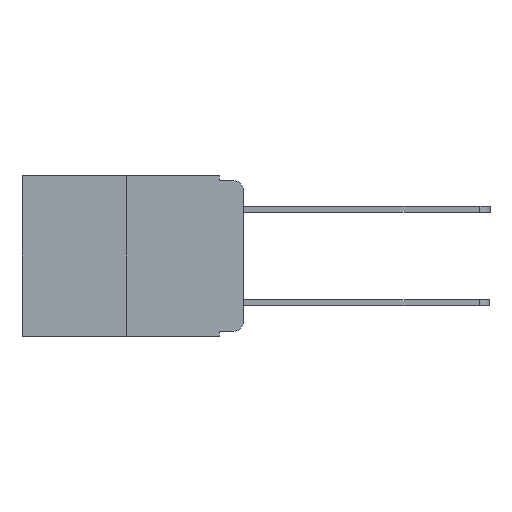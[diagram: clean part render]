
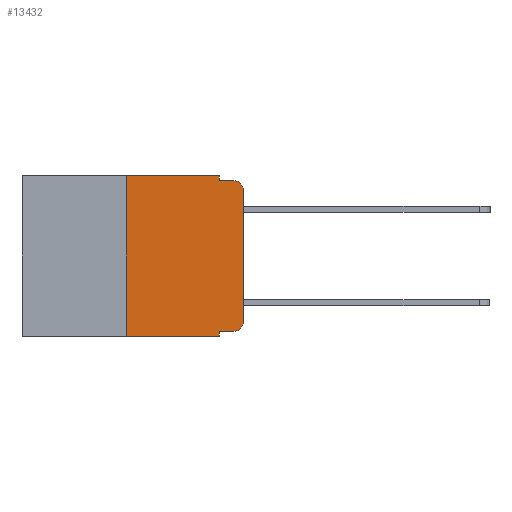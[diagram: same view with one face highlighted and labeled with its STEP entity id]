
A CAD part, left-side view. The second image highlights one B-rep face of the part: STEP entity #13432.
In plain terms, the highlighted planar face has unit normal (-1, 0, 0).
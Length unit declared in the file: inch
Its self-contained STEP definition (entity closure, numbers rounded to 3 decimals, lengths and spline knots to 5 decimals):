
#126 = CARTESIAN_POINT ( 'NONE',  ( 0., 0.051, -0.343 ) ) ;
#410 = PLANE ( 'NONE',  #3341 ) ;
#435 = EDGE_CURVE ( 'NONE', #3251, #18637, #3825, .T. ) ;
#1491 = AXIS2_PLACEMENT_3D ( 'NONE', #7417, #7707, #7675 ) ;
#1815 = EDGE_CURVE ( 'NONE', #4663, #12088, #8660, .T. ) ;
#2210 = ORIENTED_EDGE ( 'NONE', *, *, #16000, .F. ) ;
#2294 = CARTESIAN_POINT ( 'NONE',  ( 0., 0.473, 0. ) ) ;
#2514 = VECTOR ( 'NONE', #19189, 39.37008 ) ;
#3236 = LINE ( 'NONE', #6667, #21598 ) ;
#3251 = VERTEX_POINT ( 'NONE', #10124 ) ;
#3277 = DIRECTION ( 'NONE',  ( 0., 0., -1. ) ) ;
#3341 = AXIS2_PLACEMENT_3D ( 'NONE', #2294, #5998, #18486 ) ;
#3568 = FACE_OUTER_BOUND ( 'NONE', #18751, .T. ) ;
#3825 = LINE ( 'NONE', #6593, #17067 ) ;
#3938 = CARTESIAN_POINT ( 'NONE',  ( 0., 0.25, -0.343 ) ) ;
#4457 = CARTESIAN_POINT ( 'NONE',  ( 0., 0., -0.03 ) ) ;
#4663 = VERTEX_POINT ( 'NONE', #3938 ) ;
#4794 = EDGE_CURVE ( 'NONE', #7147, #11658, #18959, .T. ) ;
#5103 = EDGE_CURVE ( 'NONE', #13907, #3251, #3236, .T. ) ;
#5567 = ORIENTED_EDGE ( 'NONE', *, *, #5103, .F. ) ;
#5692 = CARTESIAN_POINT ( 'NONE',  ( 0., 0., 0. ) ) ;
#5837 = DIRECTION ( 'NONE',  ( 0., -1., 0. ) ) ;
#5998 = DIRECTION ( 'NONE',  ( 1., 0., 0. ) ) ;
#6181 = EDGE_CURVE ( 'NONE', #18637, #12114, #18896, .T. ) ;
#6483 = CARTESIAN_POINT ( 'NONE',  ( 0., 0.051, 0. ) ) ;
#6593 = CARTESIAN_POINT ( 'NONE',  ( 0., 0.051, 0. ) ) ;
#6667 = CARTESIAN_POINT ( 'NONE',  ( 0., 0.473, 0. ) ) ;
#7147 = VERTEX_POINT ( 'NONE', #16048 ) ;
#7417 = CARTESIAN_POINT ( 'NONE',  ( 0., 0.02, -0.313 ) ) ;
#7663 = CIRCLE ( 'NONE', #22209, 0.02 ) ;
#7675 = DIRECTION ( 'NONE',  ( 0., 0., -1. ) ) ;
#7707 = DIRECTION ( 'NONE',  ( -1., 0., 0. ) ) ;
#7999 = LINE ( 'NONE', #12229, #2514 ) ;
#8092 = DIRECTION ( 'NONE',  ( 0., -1., 0. ) ) ;
#8325 = ORIENTED_EDGE ( 'NONE', *, *, #10495, .T. ) ;
#8330 = CARTESIAN_POINT ( 'NONE',  ( 0., 0.02, -0.03 ) ) ;
#8633 = VECTOR ( 'NONE', #19901, 39.37008 ) ;
#8660 = LINE ( 'NONE', #13867, #22069 ) ;
#9350 = VERTEX_POINT ( 'NONE', #15884 ) ;
#9448 = EDGE_CURVE ( 'NONE', #11658, #15269, #23094, .T. ) ;
#9593 = EDGE_CURVE ( 'NONE', #4663, #13907, #19895, .T. ) ;
#9874 = CARTESIAN_POINT ( 'NONE',  ( 0., 0.051, -0.01 ) ) ;
#10124 = CARTESIAN_POINT ( 'NONE',  ( 0., 0.051, 0. ) ) ;
#10172 = DIRECTION ( 'NONE',  ( 0., 0., -1. ) ) ;
#10495 = EDGE_CURVE ( 'NONE', #9350, #7147, #7999, .T. ) ;
#11658 = VERTEX_POINT ( 'NONE', #17206 ) ;
#11831 = ORIENTED_EDGE ( 'NONE', *, *, #4794, .T. ) ;
#12032 = DIRECTION ( 'NONE',  ( 0., 0., -1. ) ) ;
#12088 = VERTEX_POINT ( 'NONE', #126 ) ;
#12114 = VERTEX_POINT ( 'NONE', #18397 ) ;
#12229 = CARTESIAN_POINT ( 'NONE',  ( 0., 0.051, -0.333 ) ) ;
#12285 = LINE ( 'NONE', #6483, #16929 ) ;
#12341 = EDGE_CURVE ( 'NONE', #15269, #12114, #7663, .T. ) ;
#13361 = DIRECTION ( 'NONE',  ( 0., 0., 1. ) ) ;
#13432 = ADVANCED_FACE ( 'NONE', ( #3568 ), #410, .F. ) ;
#13750 = ORIENTED_EDGE ( 'NONE', *, *, #9448, .T. ) ;
#13867 = CARTESIAN_POINT ( 'NONE',  ( 0., 0.473, -0.343 ) ) ;
#13907 = VERTEX_POINT ( 'NONE', #17936 ) ;
#14599 = ORIENTED_EDGE ( 'NONE', *, *, #1815, .T. ) ;
#14834 = VECTOR ( 'NONE', #13361, 39.37008 ) ;
#15081 = ORIENTED_EDGE ( 'NONE', *, *, #12341, .T. ) ;
#15269 = VERTEX_POINT ( 'NONE', #4457 ) ;
#15884 = CARTESIAN_POINT ( 'NONE',  ( 0., 0.051, -0.333 ) ) ;
#16000 = EDGE_CURVE ( 'NONE', #9350, #12088, #12285, .T. ) ;
#16048 = CARTESIAN_POINT ( 'NONE',  ( 0., 0.02, -0.333 ) ) ;
#16929 = VECTOR ( 'NONE', #12032, 39.37008 ) ;
#17067 = VECTOR ( 'NONE', #3277, 39.37008 ) ;
#17206 = CARTESIAN_POINT ( 'NONE',  ( 0., 0., -0.313 ) ) ;
#17754 = ORIENTED_EDGE ( 'NONE', *, *, #6181, .F. ) ;
#17936 = CARTESIAN_POINT ( 'NONE',  ( 0., 0.25, 0. ) ) ;
#18356 = VECTOR ( 'NONE', #8092, 39.37008 ) ;
#18397 = CARTESIAN_POINT ( 'NONE',  ( 0., 0.02, -0.01 ) ) ;
#18486 = DIRECTION ( 'NONE',  ( 0., 0., -1. ) ) ;
#18637 = VERTEX_POINT ( 'NONE', #21307 ) ;
#18751 = EDGE_LOOP ( 'NONE', ( #13750, #15081, #17754, #20945, #5567, #21174, #14599, #2210, #8325, #11831 ) ) ;
#18896 = LINE ( 'NONE', #9874, #18356 ) ;
#18959 = CIRCLE ( 'NONE', #1491, 0.02 ) ;
#19189 = DIRECTION ( 'NONE',  ( 0., -1., 0. ) ) ;
#19428 = DIRECTION ( 'NONE',  ( 0., -1., 0. ) ) ;
#19895 = LINE ( 'NONE', #21923, #14834 ) ;
#19901 = DIRECTION ( 'NONE',  ( 0., 0., 1. ) ) ;
#20612 = DIRECTION ( 'NONE',  ( -1., 0., 0. ) ) ;
#20945 = ORIENTED_EDGE ( 'NONE', *, *, #435, .F. ) ;
#21174 = ORIENTED_EDGE ( 'NONE', *, *, #9593, .F. ) ;
#21307 = CARTESIAN_POINT ( 'NONE',  ( 0., 0.051, -0.01 ) ) ;
#21598 = VECTOR ( 'NONE', #5837, 39.37008 ) ;
#21923 = CARTESIAN_POINT ( 'NONE',  ( 0., 0.25, 0. ) ) ;
#22069 = VECTOR ( 'NONE', #19428, 39.37008 ) ;
#22209 = AXIS2_PLACEMENT_3D ( 'NONE', #8330, #20612, #10172 ) ;
#23094 = LINE ( 'NONE', #5692, #8633 ) ;
